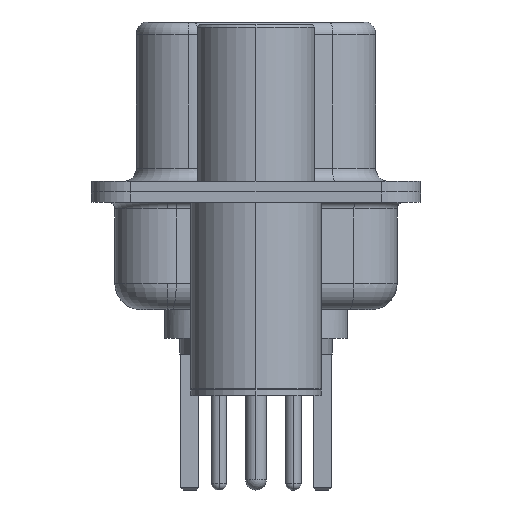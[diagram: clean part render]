
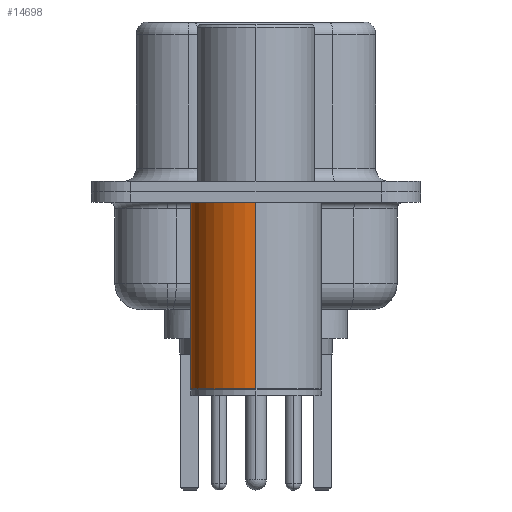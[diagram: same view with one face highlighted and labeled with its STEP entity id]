
A CAD part, left-side view. The second image highlights one B-rep face of the part: STEP entity #14698.
In plain terms, the highlighted cylindrical face has radius 2.5 mm (diameter 5 mm), a partial arc.
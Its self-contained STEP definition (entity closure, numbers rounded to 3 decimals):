
#79 = ORIENTED_EDGE ( 'NONE', *, *, #10729, .T. ) ;
#643 = CARTESIAN_POINT ( 'NONE',  ( 0., 0., 0.581 ) ) ;
#1868 = AXIS2_PLACEMENT_3D ( 'NONE', #15524, #4940, #17254 ) ;
#2061 = FACE_OUTER_BOUND ( 'NONE', #15410, .T. ) ;
#2176 = CARTESIAN_POINT ( 'NONE',  ( -2.5, 0., 0.581 ) ) ;
#2433 = DIRECTION ( 'NONE',  ( 1., 0., 0. ) ) ;
#2917 = VERTEX_POINT ( 'NONE', #11832 ) ;
#4819 = VERTEX_POINT ( 'NONE', #20399 ) ;
#4940 = DIRECTION ( 'NONE',  ( 0., 0., 1. ) ) ;
#5658 = CARTESIAN_POINT ( 'NONE',  ( 0., 0., -0.4 ) ) ;
#5950 = VERTEX_POINT ( 'NONE', #19993 ) ;
#6162 = CYLINDRICAL_SURFACE ( 'NONE', #21217, 2.5 ) ;
#6332 = CIRCLE ( 'NONE', #12112, 2.5 ) ;
#6489 = DIRECTION ( 'NONE',  ( 0., 0., 1. ) ) ;
#7394 = DIRECTION ( 'NONE',  ( 1., 0., 0. ) ) ;
#8209 = CARTESIAN_POINT ( 'NONE',  ( 2.5, 0., 0.581 ) ) ;
#9018 = CIRCLE ( 'NONE', #1868, 2.5 ) ;
#10237 = EDGE_CURVE ( 'NONE', #2917, #4819, #19967, .T. ) ;
#10729 = EDGE_CURVE ( 'NONE', #5950, #11557, #19950, .T. ) ;
#11322 = ORIENTED_EDGE ( 'NONE', *, *, #17273, .F. ) ;
#11557 = VERTEX_POINT ( 'NONE', #12226 ) ;
#11832 = CARTESIAN_POINT ( 'NONE',  ( 2.5, 0., -7.525 ) ) ;
#12112 = AXIS2_PLACEMENT_3D ( 'NONE', #5658, #17970, #7394 ) ;
#12226 = CARTESIAN_POINT ( 'NONE',  ( -2.5, 0., -0.4 ) ) ;
#14698 = ADVANCED_FACE ( 'NONE', ( #2061 ), #6162, .T. ) ;
#14720 = DIRECTION ( 'NONE',  ( 0., 0., 1. ) ) ;
#14776 = VECTOR ( 'NONE', #6489, 1000. ) ;
#15410 = EDGE_LOOP ( 'NONE', ( #19215, #79, #11322, #19038 ) ) ;
#15524 = CARTESIAN_POINT ( 'NONE',  ( 0., 0., -7.525 ) ) ;
#17254 = DIRECTION ( 'NONE',  ( 1., 0., 0. ) ) ;
#17273 = EDGE_CURVE ( 'NONE', #4819, #11557, #6332, .T. ) ;
#17678 = EDGE_CURVE ( 'NONE', #2917, #5950, #9018, .T. ) ;
#17970 = DIRECTION ( 'NONE',  ( 0., 0., 1. ) ) ;
#19038 = ORIENTED_EDGE ( 'NONE', *, *, #10237, .F. ) ;
#19215 = ORIENTED_EDGE ( 'NONE', *, *, #17678, .T. ) ;
#19950 = LINE ( 'NONE', #2176, #20484 ) ;
#19967 = LINE ( 'NONE', #8209, #14776 ) ;
#19993 = CARTESIAN_POINT ( 'NONE',  ( -2.5, 0., -7.525 ) ) ;
#20399 = CARTESIAN_POINT ( 'NONE',  ( 2.5, 0., -0.4 ) ) ;
#20484 = VECTOR ( 'NONE', #21429, 1000. ) ;
#21217 = AXIS2_PLACEMENT_3D ( 'NONE', #643, #14720, #2433 ) ;
#21429 = DIRECTION ( 'NONE',  ( 0., 0., 1. ) ) ;
